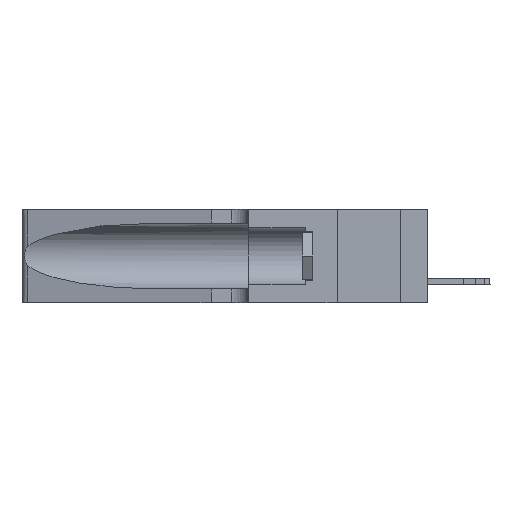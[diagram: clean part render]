
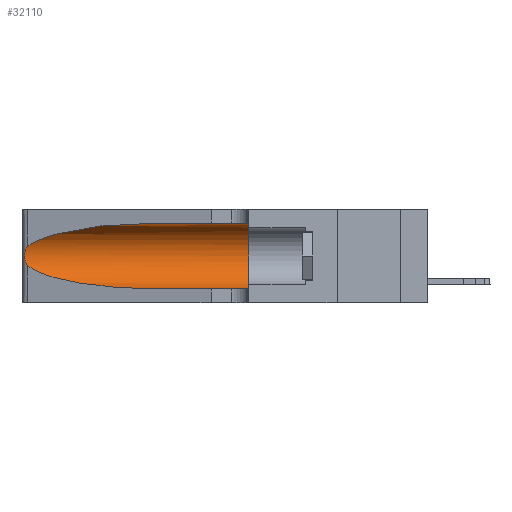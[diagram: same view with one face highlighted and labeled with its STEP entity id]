
A CAD part, left-side view. The second image highlights one B-rep face of the part: STEP entity #32110.
In plain terms, the highlighted cylindrical face has radius 3.308 mm (diameter 6.617 mm), a partial arc.
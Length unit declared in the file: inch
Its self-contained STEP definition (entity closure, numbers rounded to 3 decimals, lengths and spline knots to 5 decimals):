
#277 = VECTOR ( 'NONE', #27223, 39.37008 ) ;
#362 = CARTESIAN_POINT ( 'NONE',  ( 0.18966, 0.96281, 0.31525 ) ) ;
#793 = FACE_OUTER_BOUND ( 'NONE', #27781, .T. ) ;
#1357 = EDGE_CURVE ( 'NONE', #13905, #3677, #24503, .T. ) ;
#3001 = CARTESIAN_POINT ( 'NONE',  ( 0.25487, 1.22718, 0.22369 ) ) ;
#3458 = CARTESIAN_POINT ( 'NONE',  ( 0.25555, 1.22993, 0.14849 ) ) ;
#3677 = VERTEX_POINT ( 'NONE', #28673 ) ;
#3971 = ORIENTED_EDGE ( 'NONE', *, *, #20422, .T. ) ;
#4140 = B_SPLINE_CURVE_WITH_KNOTS ( 'NONE', 3,
 ( #17080, #22144, #22269, #27568, #14144, #11351, #30273, #19621, #6042, #27690, #19744, #16942, #3458, #6282 ),
 .UNSPECIFIED., .F., .F.,
 ( 4, 2, 2, 2, 2, 2, 4 ),
 ( 0., 0.00027, 0.00053, 0.00107, 0.0016, 0.00187, 0.00214 ),
 .UNSPECIFIED. ) ;
#5294 = CARTESIAN_POINT ( 'NONE',  ( 0.25487, 1.22718, 0.14631 ) ) ;
#5460 = DIRECTION ( 'NONE',  ( 0., -1., 0. ) ) ;
#6042 = CARTESIAN_POINT ( 'NONE',  ( 0.26017, 1.23833, 0.17102 ) ) ;
#6145 = CARTESIAN_POINT ( 'NONE',  ( 0.18966, 0.96281, 0.05475 ) ) ;
#6282 = CARTESIAN_POINT ( 'NONE',  ( 0.25487, 1.22718, 0.14631 ) ) ;
#7517 = LINE ( 'NONE', #12911, #277 ) ;
#9360 = DIRECTION ( 'NONE',  ( 0., 0., 1. ) ) ;
#9620 = CARTESIAN_POINT ( 'NONE',  ( 0.1305, 1.61858, 0.05475 ) ) ;
#9687 = CYLINDRICAL_SURFACE ( 'NONE', #20389, 0.13025 ) ;
#10187 = EDGE_CURVE ( 'NONE', #27466, #28009, #11285, .T. ) ;
#10917 = VECTOR ( 'NONE', #23261, 39.37008 ) ;
#11285 = CIRCLE ( 'NONE', #25177, 0.13025 ) ;
#11351 = CARTESIAN_POINT ( 'NONE',  ( 0.26018, 1.23835, 0.19895 ) ) ;
#12911 = CARTESIAN_POINT ( 'NONE',  ( 0.1305, 1.61858, 0.31525 ) ) ;
#13030 = VERTEX_POINT ( 'NONE', #26985 ) ;
#13905 = VERTEX_POINT ( 'NONE', #15970 ) ;
#14144 = CARTESIAN_POINT ( 'NONE',  ( 0.25854, 1.2359, 0.20912 ) ) ;
#14638 = CARTESIAN_POINT ( 'NONE',  ( 0.1305, 0.35, 0.185 ) ) ;
#15598 =( BOUNDED_CURVE ( )  B_SPLINE_CURVE ( 3, ( #33168, #362, #25112, #3001 ),
 .UNSPECIFIED., .F., .T. ) 
 B_SPLINE_CURVE_WITH_KNOTS ( ( 4, 4 ),
 ( 1.5708, 2.84003 ),
 .UNSPECIFIED. ) 
 CURVE ( )  GEOMETRIC_REPRESENTATION_ITEM ( )  RATIONAL_B_SPLINE_CURVE ( ( 1., 0.87, 0.87, 1. ) ) 
 REPRESENTATION_ITEM ( '' )  );
#15676 = ORIENTED_EDGE ( 'NONE', *, *, #1357, .T. ) ;
#15970 = CARTESIAN_POINT ( 'NONE',  ( 0.25487, 1.22718, 0.14631 ) ) ;
#16942 = CARTESIAN_POINT ( 'NONE',  ( 0.25639, 1.23186, 0.15144 ) ) ;
#17080 = CARTESIAN_POINT ( 'NONE',  ( 0.25487, 1.22718, 0.22369 ) ) ;
#18430 = ORIENTED_EDGE ( 'NONE', *, *, #10187, .F. ) ;
#19621 = CARTESIAN_POINT ( 'NONE',  ( 0.26075, 1.23896, 0.178 ) ) ;
#19744 = CARTESIAN_POINT ( 'NONE',  ( 0.25789, 1.23486, 0.15765 ) ) ;
#19845 = CARTESIAN_POINT ( 'NONE',  ( 0.1305, 0.72297, 0.05475 ) ) ;
#20116 = DIRECTION ( 'NONE',  ( 0., 1., 0. ) ) ;
#20389 = AXIS2_PLACEMENT_3D ( 'NONE', #32198, #5460, #27101 ) ;
#20422 = EDGE_CURVE ( 'NONE', #13030, #13905, #4140, .T. ) ;
#21201 = ORIENTED_EDGE ( 'NONE', *, *, #32790, .F. ) ;
#21229 = CARTESIAN_POINT ( 'NONE',  ( 0.2373, 1.15595, 0.08982 ) ) ;
#21766 = ORIENTED_EDGE ( 'NONE', *, *, #34008, .T. ) ;
#21917 = LINE ( 'NONE', #9620, #10917 ) ;
#22144 = CARTESIAN_POINT ( 'NONE',  ( 0.25555, 1.22994, 0.2215 ) ) ;
#22269 = CARTESIAN_POINT ( 'NONE',  ( 0.25639, 1.23184, 0.21858 ) ) ;
#23261 = DIRECTION ( 'NONE',  ( 0., -1., 0. ) ) ;
#23445 = CARTESIAN_POINT ( 'NONE',  ( 0.1305, 0.35, 0.31525 ) ) ;
#24503 =( BOUNDED_CURVE ( )  B_SPLINE_CURVE ( 3, ( #5294, #21229, #6145, #19845 ),
 .UNSPECIFIED., .F., .F. ) 
 B_SPLINE_CURVE_WITH_KNOTS ( ( 4, 4 ),
 ( 3.44316, 4.71239 ),
 .UNSPECIFIED. ) 
 CURVE ( )  GEOMETRIC_REPRESENTATION_ITEM ( )  RATIONAL_B_SPLINE_CURVE ( ( 1., 0.87, 0.87, 1. ) ) 
 REPRESENTATION_ITEM ( '' )  );
#25112 = CARTESIAN_POINT ( 'NONE',  ( 0.2373, 1.15595, 0.28018 ) ) ;
#25177 = AXIS2_PLACEMENT_3D ( 'NONE', #14638, #20116, #9360 ) ;
#25427 = VERTEX_POINT ( 'NONE', #29278 ) ;
#26985 = CARTESIAN_POINT ( 'NONE',  ( 0.25487, 1.22718, 0.22369 ) ) ;
#27101 = DIRECTION ( 'NONE',  ( 0., 0., -1. ) ) ;
#27223 = DIRECTION ( 'NONE',  ( 0., -1., 0. ) ) ;
#27466 = VERTEX_POINT ( 'NONE', #23445 ) ;
#27568 = CARTESIAN_POINT ( 'NONE',  ( 0.25787, 1.23484, 0.2124 ) ) ;
#27690 = CARTESIAN_POINT ( 'NONE',  ( 0.25856, 1.23593, 0.16098 ) ) ;
#27781 = EDGE_LOOP ( 'NONE', ( #31120, #3971, #15676, #21766, #18430, #21201 ) ) ;
#28009 = VERTEX_POINT ( 'NONE', #31357 ) ;
#28673 = CARTESIAN_POINT ( 'NONE',  ( 0.1305, 0.72297, 0.05475 ) ) ;
#29278 = CARTESIAN_POINT ( 'NONE',  ( 0.1305, 0.72297, 0.31525 ) ) ;
#29430 = EDGE_CURVE ( 'NONE', #25427, #13030, #15598, .T. ) ;
#30273 = CARTESIAN_POINT ( 'NONE',  ( 0.26075, 1.23896, 0.19203 ) ) ;
#31120 = ORIENTED_EDGE ( 'NONE', *, *, #29430, .T. ) ;
#31357 = CARTESIAN_POINT ( 'NONE',  ( 0.1305, 0.35, 0.05475 ) ) ;
#32110 = ADVANCED_FACE ( 'NONE', ( #793 ), #9687, .F. ) ;
#32198 = CARTESIAN_POINT ( 'NONE',  ( 0.1305, 1.61858, 0.185 ) ) ;
#32790 = EDGE_CURVE ( 'NONE', #25427, #27466, #7517, .T. ) ;
#33168 = CARTESIAN_POINT ( 'NONE',  ( 0.1305, 0.72297, 0.31525 ) ) ;
#34008 = EDGE_CURVE ( 'NONE', #3677, #28009, #21917, .T. ) ;
